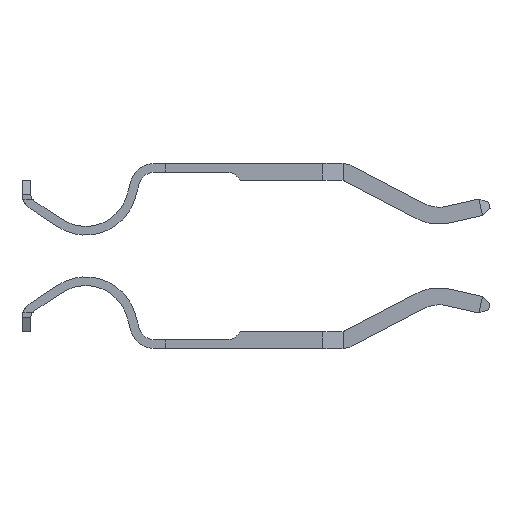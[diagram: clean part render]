
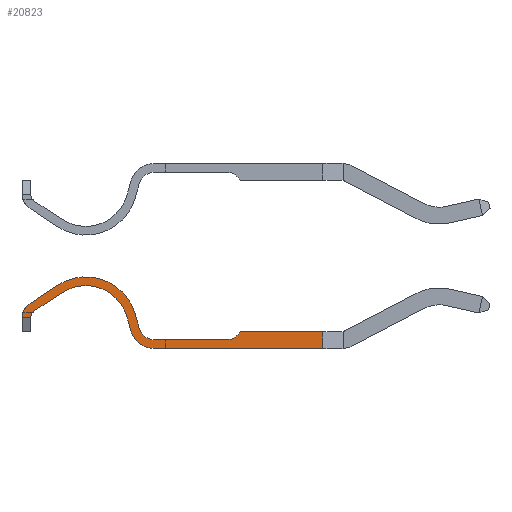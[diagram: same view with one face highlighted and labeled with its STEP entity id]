
A CAD part, left-side view. The second image highlights one B-rep face of the part: STEP entity #20823.
In plain terms, the highlighted face is planar.
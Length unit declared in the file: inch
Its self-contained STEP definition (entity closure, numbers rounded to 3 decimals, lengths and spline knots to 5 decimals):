
#8 = CARTESIAN_POINT ( 'NONE',  ( 0.33, 0.0125, 0.025 ) ) ;
#98 = AXIS2_PLACEMENT_3D ( 'NONE', #14640, #878, #17001 ) ;
#151 = DIRECTION ( 'NONE',  ( 1., 0., 0. ) ) ;
#169 = LINE ( 'NONE', #5114, #23948 ) ;
#504 = EDGE_CURVE ( 'NONE', #9163, #16431, #7479, .T. ) ;
#678 = EDGE_CURVE ( 'NONE', #7638, #24248, #16405, .T. ) ;
#878 = DIRECTION ( 'NONE',  ( 0., 0., -1. ) ) ;
#888 = DIRECTION ( 'NONE',  ( 1., 0., 0. ) ) ;
#956 = ORIENTED_EDGE ( 'NONE', *, *, #4874, .T. ) ;
#1229 = ORIENTED_EDGE ( 'NONE', *, *, #25357, .F. ) ;
#1466 = CARTESIAN_POINT ( 'NONE',  ( 0.43721, 0.04723, 0.025 ) ) ;
#1543 = VECTOR ( 'NONE', #13864, 39.37008 ) ;
#1576 = ORIENTED_EDGE ( 'NONE', *, *, #10382, .F. ) ;
#1891 = VERTEX_POINT ( 'NONE', #8067 ) ;
#2158 = CARTESIAN_POINT ( 'NONE',  ( 0.43721, 0.0255, 0.025 ) ) ;
#2166 = LINE ( 'NONE', #18421, #25908 ) ;
#2755 = ORIENTED_EDGE ( 'NONE', *, *, #4007, .T. ) ;
#3008 = LINE ( 'NONE', #8, #1543 ) ;
#3277 = CARTESIAN_POINT ( 'NONE',  ( 0.15971, 0.0575, 0.025 ) ) ;
#3348 = AXIS2_PLACEMENT_3D ( 'NONE', #27729, #13907, #151 ) ;
#3379 = CARTESIAN_POINT ( 'NONE',  ( 0.18604, 0.10646, 0.025 ) ) ;
#3653 = VERTEX_POINT ( 'NONE', #7278 ) ;
#3769 = ORIENTED_EDGE ( 'NONE', *, *, #14135, .F. ) ;
#3801 = DIRECTION ( 'NONE',  ( 1., 0., 0. ) ) ;
#3891 = CIRCLE ( 'NONE', #3348, 0.0235 ) ;
#3973 = VERTEX_POINT ( 'NONE', #14026 ) ;
#4007 = EDGE_CURVE ( 'NONE', #3973, #25213, #13688, .T. ) ;
#4015 = EDGE_CURVE ( 'NONE', #27847, #25985, #25963, .T. ) ;
#4307 = CARTESIAN_POINT ( 'NONE',  ( 0.33, 0.0255, 0.025 ) ) ;
#4874 = EDGE_CURVE ( 'NONE', #8705, #10379, #13632, .T. ) ;
#4973 = CARTESIAN_POINT ( 'NONE',  ( 0.45258, 0.03186, 0.025 ) ) ;
#5114 = CARTESIAN_POINT ( 'NONE',  ( 0.45821, 0.0375, 0.025 ) ) ;
#5213 = CARTESIAN_POINT ( 'NONE',  ( 0.228, 0.0425, 0.025 ) ) ;
#5540 = DIRECTION ( 'NONE',  ( -1., 0., 0. ) ) ;
#5840 = ORIENTED_EDGE ( 'NONE', *, *, #14187, .T. ) ;
#5899 = CARTESIAN_POINT ( 'NONE',  ( 0.14518, 0.07966, 0.025 ) ) ;
#6088 = VERTEX_POINT ( 'NONE', #21392 ) ;
#6510 = CARTESIAN_POINT ( 'NONE',  ( 0.28917, 0.05955, 0.025 ) ) ;
#7278 = CARTESIAN_POINT ( 'NONE',  ( 0.58021, 0.0375, 0.025 ) ) ;
#7479 = CIRCLE ( 'NONE', #12747, 0.0365 ) ;
#7502 = DIRECTION ( 'NONE',  ( -1., 0., 0. ) ) ;
#7574 = EDGE_CURVE ( 'NONE', #10379, #9163, #23814, .T. ) ;
#7638 = VERTEX_POINT ( 'NONE', #11324 ) ;
#7806 = VECTOR ( 'NONE', #11209, 39.37008 ) ;
#8067 = CARTESIAN_POINT ( 'NONE',  ( 0.58021, 0.0125, 0.025 ) ) ;
#8135 = CIRCLE ( 'NONE', #20730, 0.0765 ) ;
#8313 = DIRECTION ( 'NONE',  ( 0., 0., 1. ) ) ;
#8705 = VERTEX_POINT ( 'NONE', #24404 ) ;
#8732 = DIRECTION ( 'NONE',  ( 0.836, 0.549, 0. ) ) ;
#9041 = VECTOR ( 'NONE', #10030, 39.37008 ) ;
#9082 = ORIENTED_EDGE ( 'NONE', *, *, #678, .T. ) ;
#9163 = VERTEX_POINT ( 'NONE', #28178 ) ;
#9252 = DIRECTION ( 'NONE',  ( 0.836, 0.549, 0. ) ) ;
#9291 = DIRECTION ( 'NONE',  ( 1., 0., 0. ) ) ;
#9559 = DIRECTION ( 'NONE',  ( 1., 0., 0. ) ) ;
#10030 = DIRECTION ( 'NONE',  ( -0.707, -0.707, 0. ) ) ;
#10371 = EDGE_CURVE ( 'NONE', #12254, #26295, #24287, .T. ) ;
#10379 = VERTEX_POINT ( 'NONE', #11489 ) ;
#10382 = EDGE_CURVE ( 'NONE', #20369, #12254, #3891, .T. ) ;
#10470 = ORIENTED_EDGE ( 'NONE', *, *, #23702, .T. ) ;
#10739 = PLANE ( 'NONE',  #26383 ) ;
#11209 = DIRECTION ( 'NONE',  ( 0.268, -0.963, 0. ) ) ;
#11324 = CARTESIAN_POINT ( 'NONE',  ( 0.13322, 0.058, 0.025 ) ) ;
#11489 = CARTESIAN_POINT ( 'NONE',  ( 0.28917, 0.05955, 0.025 ) ) ;
#11520 = VECTOR ( 'NONE', #15794, 39.37008 ) ;
#11824 = EDGE_CURVE ( 'NONE', #3653, #3973, #169, .T. ) ;
#12011 = CARTESIAN_POINT ( 'NONE',  ( 0.58021, 0.0375, 0.025 ) ) ;
#12030 = AXIS2_PLACEMENT_3D ( 'NONE', #12773, #28873, #15111 ) ;
#12254 = VERTEX_POINT ( 'NONE', #4307 ) ;
#12747 = AXIS2_PLACEMENT_3D ( 'NONE', #28957, #8313, #9291 ) ;
#12773 = CARTESIAN_POINT ( 'NONE',  ( 0.228, 0.0425, 0.025 ) ) ;
#12865 = ORIENTED_EDGE ( 'NONE', *, *, #7574, .T. ) ;
#13051 = DIRECTION ( 'NONE',  ( 0., 0., -1. ) ) ;
#13122 = CARTESIAN_POINT ( 'NONE',  ( 0.33, 0.0125, 0.025 ) ) ;
#13382 = CARTESIAN_POINT ( 'NONE',  ( 0.14621, 0.058, 0.025 ) ) ;
#13632 = CIRCLE ( 'NONE', #12030, 0.0635 ) ;
#13688 = LINE ( 'NONE', #24588, #9041 ) ;
#13864 = DIRECTION ( 'NONE',  ( 1., 0., 0. ) ) ;
#13907 = DIRECTION ( 'NONE',  ( 0., 0., 1. ) ) ;
#14026 = CARTESIAN_POINT ( 'NONE',  ( 0.45821, 0.0375, 0.025 ) ) ;
#14135 = EDGE_CURVE ( 'NONE', #25985, #19957, #8135, .T. ) ;
#14187 = EDGE_CURVE ( 'NONE', #24248, #6088, #23641, .T. ) ;
#14334 = DIRECTION ( 'NONE',  ( -1., 0., 0. ) ) ;
#14640 = CARTESIAN_POINT ( 'NONE',  ( 0.15971, 0.0575, 0.025 ) ) ;
#15111 = DIRECTION ( 'NONE',  ( -1., 0., 0. ) ) ;
#15403 = ORIENTED_EDGE ( 'NONE', *, *, #11824, .T. ) ;
#15491 = AXIS2_PLACEMENT_3D ( 'NONE', #1466, #17567, #3801 ) ;
#15794 = DIRECTION ( 'NONE',  ( 0.268, -0.963, 0. ) ) ;
#15850 = AXIS2_PLACEMENT_3D ( 'NONE', #3277, #19355, #5540 ) ;
#16291 = ORIENTED_EDGE ( 'NONE', *, *, #27023, .F. ) ;
#16405 = LINE ( 'NONE', #13382, #21790 ) ;
#16431 = VERTEX_POINT ( 'NONE', #13122 ) ;
#16833 = FACE_OUTER_BOUND ( 'NONE', #27764, .T. ) ;
#16968 = CARTESIAN_POINT ( 'NONE',  ( 0.30169, 0.06304, 0.025 ) ) ;
#17001 = DIRECTION ( 'NONE',  ( -1., 0., 0. ) ) ;
#17567 = DIRECTION ( 'NONE',  ( 0., 0., -1. ) ) ;
#17667 = ORIENTED_EDGE ( 'NONE', *, *, #10371, .F. ) ;
#18152 = VECTOR ( 'NONE', #888, 39.37008 ) ;
#18421 = CARTESIAN_POINT ( 'NONE',  ( 0.15231, 0.06879, 0.025 ) ) ;
#18969 = LINE ( 'NONE', #12011, #24381 ) ;
#19160 = CARTESIAN_POINT ( 'NONE',  ( 0.14518, 0.07966, 0.025 ) ) ;
#19293 = EDGE_CURVE ( 'NONE', #6088, #8705, #2166, .T. ) ;
#19338 = CIRCLE ( 'NONE', #15491, 0.02173 ) ;
#19355 = DIRECTION ( 'NONE',  ( 0., 0., -1. ) ) ;
#19957 = VERTEX_POINT ( 'NONE', #16968 ) ;
#20279 = ORIENTED_EDGE ( 'NONE', *, *, #21219, .F. ) ;
#20369 = VERTEX_POINT ( 'NONE', #20666 ) ;
#20417 = CARTESIAN_POINT ( 'NONE',  ( 0.30169, 0.06304, 0.025 ) ) ;
#20666 = CARTESIAN_POINT ( 'NONE',  ( 0.30736, 0.04269, 0.025 ) ) ;
#20730 = AXIS2_PLACEMENT_3D ( 'NONE', #5213, #21311, #7502 ) ;
#20823 = ADVANCED_FACE ( 'NONE', ( #16833 ), #10739, .F. ) ;
#21219 = EDGE_CURVE ( 'NONE', #3653, #1891, #18969, .T. ) ;
#21311 = DIRECTION ( 'NONE',  ( 0., 0., -1. ) ) ;
#21392 = CARTESIAN_POINT ( 'NONE',  ( 0.15231, 0.06879, 0.025 ) ) ;
#21790 = VECTOR ( 'NONE', #9559, 39.37008 ) ;
#22593 = ORIENTED_EDGE ( 'NONE', *, *, #27518, .T. ) ;
#23346 = ORIENTED_EDGE ( 'NONE', *, *, #4015, .F. ) ;
#23544 = DIRECTION ( 'NONE',  ( 0., -1., 0. ) ) ;
#23641 = CIRCLE ( 'NONE', #98, 0.0135 ) ;
#23702 = EDGE_CURVE ( 'NONE', #16431, #1891, #3008, .T. ) ;
#23814 = LINE ( 'NONE', #6510, #11520 ) ;
#23948 = VECTOR ( 'NONE', #14334, 39.37008 ) ;
#24248 = VERTEX_POINT ( 'NONE', #24761 ) ;
#24287 = LINE ( 'NONE', #28447, #18152 ) ;
#24381 = VECTOR ( 'NONE', #23544, 39.37008 ) ;
#24404 = CARTESIAN_POINT ( 'NONE',  ( 0.19317, 0.09559, 0.025 ) ) ;
#24574 = CARTESIAN_POINT ( 'NONE',  ( 0.095, 0.025, 0.025 ) ) ;
#24588 = CARTESIAN_POINT ( 'NONE',  ( 0.45821, 0.0375, 0.025 ) ) ;
#24761 = CARTESIAN_POINT ( 'NONE',  ( 0.14622, 0.058, 0.025 ) ) ;
#25213 = VERTEX_POINT ( 'NONE', #4973 ) ;
#25267 = VECTOR ( 'NONE', #8732, 39.37008 ) ;
#25277 = CIRCLE ( 'NONE', #15850, 0.0265 ) ;
#25357 = EDGE_CURVE ( 'NONE', #7638, #27847, #25277, .T. ) ;
#25908 = VECTOR ( 'NONE', #9252, 39.37008 ) ;
#25963 = LINE ( 'NONE', #5899, #25267 ) ;
#25985 = VERTEX_POINT ( 'NONE', #3379 ) ;
#26204 = LINE ( 'NONE', #20417, #7806 ) ;
#26295 = VERTEX_POINT ( 'NONE', #2158 ) ;
#26356 = ORIENTED_EDGE ( 'NONE', *, *, #504, .T. ) ;
#26383 = AXIS2_PLACEMENT_3D ( 'NONE', #24574, #13051, #29133 ) ;
#27023 = EDGE_CURVE ( 'NONE', #19957, #20369, #26204, .T. ) ;
#27518 = EDGE_CURVE ( 'NONE', #25213, #26295, #19338, .T. ) ;
#27729 = CARTESIAN_POINT ( 'NONE',  ( 0.33, 0.049, 0.025 ) ) ;
#27764 = EDGE_LOOP ( 'NONE', ( #1229, #9082, #5840, #29049, #956, #12865, #26356, #10470, #20279, #15403, #2755, #22593, #17667, #1576, #16291, #3769, #23346 ) ) ;
#27847 = VERTEX_POINT ( 'NONE', #19160 ) ;
#28178 = CARTESIAN_POINT ( 'NONE',  ( 0.29484, 0.0392, 0.025 ) ) ;
#28447 = CARTESIAN_POINT ( 'NONE',  ( 0.33, 0.0255, 0.025 ) ) ;
#28873 = DIRECTION ( 'NONE',  ( 0., 0., -1. ) ) ;
#28957 = CARTESIAN_POINT ( 'NONE',  ( 0.33, 0.049, 0.025 ) ) ;
#29049 = ORIENTED_EDGE ( 'NONE', *, *, #19293, .T. ) ;
#29133 = DIRECTION ( 'NONE',  ( -1., 0., 0. ) ) ;
